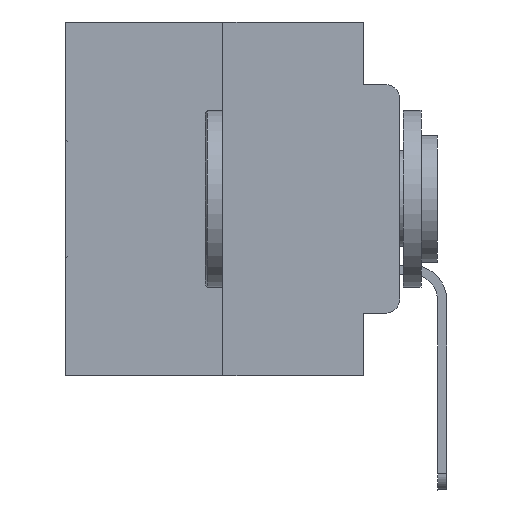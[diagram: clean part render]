
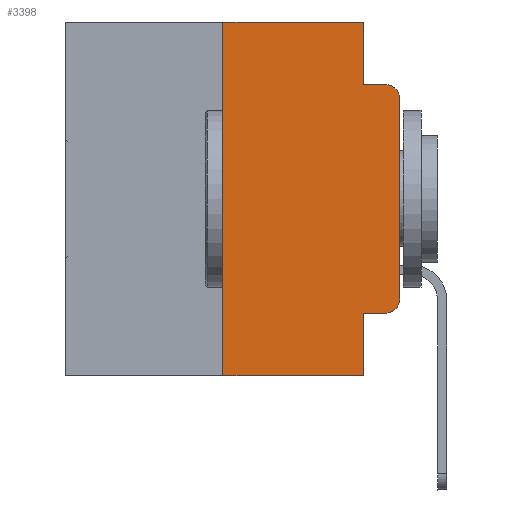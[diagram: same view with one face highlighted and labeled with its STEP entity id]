
A CAD part, left-side view. The second image highlights one B-rep face of the part: STEP entity #3398.
In plain terms, the highlighted planar face has unit normal (-1, 0, 0).
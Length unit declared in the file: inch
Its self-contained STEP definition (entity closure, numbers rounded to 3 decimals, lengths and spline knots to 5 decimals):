
#674 = DIRECTION ( 'NONE',  ( -1., 0., 0. ) ) ;
#1732 = EDGE_CURVE ( 'NONE', #10366, #27872, #18274, .T. ) ;
#1912 = VERTEX_POINT ( 'NONE', #21040 ) ;
#2130 = EDGE_CURVE ( 'NONE', #7641, #21543, #20553, .T. ) ;
#2173 = DIRECTION ( 'NONE',  ( 0., 0., -1. ) ) ;
#2316 = CARTESIAN_POINT ( 'NONE',  ( 0., 0.473, 0. ) ) ;
#2382 = VECTOR ( 'NONE', #18205, 39.37008 ) ;
#2427 = ORIENTED_EDGE ( 'NONE', *, *, #14850, .F. ) ;
#2799 = ORIENTED_EDGE ( 'NONE', *, *, #20841, .T. ) ;
#3170 = AXIS2_PLACEMENT_3D ( 'NONE', #11719, #674, #25266 ) ;
#3317 = CARTESIAN_POINT ( 'NONE',  ( 0., 0., 0. ) ) ;
#3398 = ADVANCED_FACE ( 'NONE', ( #11137 ), #13498, .F. ) ;
#4676 = EDGE_CURVE ( 'NONE', #13734, #19552, #22344, .T. ) ;
#5576 = ORIENTED_EDGE ( 'NONE', *, *, #4676, .F. ) ;
#5836 = VERTEX_POINT ( 'NONE', #7557 ) ;
#6336 = CARTESIAN_POINT ( 'NONE',  ( 0., 0.051, 0. ) ) ;
#6423 = DIRECTION ( 'NONE',  ( 0., -1., 0. ) ) ;
#6621 = CARTESIAN_POINT ( 'NONE',  ( 0., 0.02, -0.1085 ) ) ;
#6724 = CARTESIAN_POINT ( 'NONE',  ( 0., 0.25, 0. ) ) ;
#6899 = DIRECTION ( 'NONE',  ( -1., 0., 0. ) ) ;
#7078 = DIRECTION ( 'NONE',  ( 0., -1., 0. ) ) ;
#7557 = CARTESIAN_POINT ( 'NONE',  ( 0., 0., -0.3915 ) ) ;
#7641 = VERTEX_POINT ( 'NONE', #23412 ) ;
#7825 = LINE ( 'NONE', #10033, #12091 ) ;
#9768 = CARTESIAN_POINT ( 'NONE',  ( 0., 0., -0.1085 ) ) ;
#9896 = DIRECTION ( 'NONE',  ( 0., 0., -1. ) ) ;
#10033 = CARTESIAN_POINT ( 'NONE',  ( 0., 0.051, 0. ) ) ;
#10095 = ORIENTED_EDGE ( 'NONE', *, *, #27445, .F. ) ;
#10366 = VERTEX_POINT ( 'NONE', #9768 ) ;
#11137 = FACE_OUTER_BOUND ( 'NONE', #25460, .T. ) ;
#11202 = VECTOR ( 'NONE', #6423, 39.37008 ) ;
#11481 = CARTESIAN_POINT ( 'NONE',  ( 0., 0.473, -0.5 ) ) ;
#11497 = CARTESIAN_POINT ( 'NONE',  ( 0., 0.25, 0. ) ) ;
#11633 = CARTESIAN_POINT ( 'NONE',  ( 0., 0.051, -0.0885 ) ) ;
#11719 = CARTESIAN_POINT ( 'NONE',  ( 0., 0.02, -0.3915 ) ) ;
#11766 = CARTESIAN_POINT ( 'NONE',  ( 0., 0.051, -0.4115 ) ) ;
#12091 = VECTOR ( 'NONE', #9896, 39.37008 ) ;
#13355 = DIRECTION ( 'NONE',  ( 0., 0., -1. ) ) ;
#13498 = PLANE ( 'NONE',  #20268 ) ;
#13734 = VERTEX_POINT ( 'NONE', #15559 ) ;
#13778 = EDGE_CURVE ( 'NONE', #1912, #5836, #20082, .T. ) ;
#13835 = ORIENTED_EDGE ( 'NONE', *, *, #24456, .T. ) ;
#14768 = DIRECTION ( 'NONE',  ( 0., 0., 1. ) ) ;
#14850 = EDGE_CURVE ( 'NONE', #21543, #27362, #27032, .T. ) ;
#15559 = CARTESIAN_POINT ( 'NONE',  ( 0., 0.051, -0.4115 ) ) ;
#15654 = ORIENTED_EDGE ( 'NONE', *, *, #25954, .F. ) ;
#15881 = LINE ( 'NONE', #11766, #17844 ) ;
#16478 = DIRECTION ( 'NONE',  ( 0., -1., 0. ) ) ;
#16547 = ORIENTED_EDGE ( 'NONE', *, *, #13778, .T. ) ;
#16866 = VECTOR ( 'NONE', #20192, 39.37008 ) ;
#17844 = VECTOR ( 'NONE', #16478, 39.37008 ) ;
#18205 = DIRECTION ( 'NONE',  ( 0., 0., 1. ) ) ;
#18213 = CARTESIAN_POINT ( 'NONE',  ( 0., 0.473, 0. ) ) ;
#18274 = CIRCLE ( 'NONE', #27205, 0.02 ) ;
#18275 = LINE ( 'NONE', #11633, #16866 ) ;
#19164 = VECTOR ( 'NONE', #14768, 39.37008 ) ;
#19552 = VERTEX_POINT ( 'NONE', #25103 ) ;
#20026 = LINE ( 'NONE', #11481, #22937 ) ;
#20082 = CIRCLE ( 'NONE', #3170, 0.02 ) ;
#20107 = ORIENTED_EDGE ( 'NONE', *, *, #1732, .T. ) ;
#20192 = DIRECTION ( 'NONE',  ( 0., -1., 0. ) ) ;
#20268 = AXIS2_PLACEMENT_3D ( 'NONE', #18213, #22489, #13355 ) ;
#20553 = LINE ( 'NONE', #6724, #2382 ) ;
#20782 = ORIENTED_EDGE ( 'NONE', *, *, #26196, .T. ) ;
#20841 = EDGE_CURVE ( 'NONE', #13734, #1912, #15881, .T. ) ;
#20945 = CARTESIAN_POINT ( 'NONE',  ( 0., 0.051, -0.0885 ) ) ;
#21040 = CARTESIAN_POINT ( 'NONE',  ( 0., 0.02, -0.4115 ) ) ;
#21543 = VERTEX_POINT ( 'NONE', #11497 ) ;
#21691 = ORIENTED_EDGE ( 'NONE', *, *, #2130, .F. ) ;
#21905 = CARTESIAN_POINT ( 'NONE',  ( 0., 0.051, 0. ) ) ;
#22344 = LINE ( 'NONE', #21905, #24574 ) ;
#22489 = DIRECTION ( 'NONE',  ( 1., 0., 0. ) ) ;
#22937 = VECTOR ( 'NONE', #7078, 39.37008 ) ;
#23412 = CARTESIAN_POINT ( 'NONE',  ( 0., 0.25, -0.5 ) ) ;
#23478 = LINE ( 'NONE', #3317, #19164 ) ;
#24456 = EDGE_CURVE ( 'NONE', #5836, #10366, #23478, .T. ) ;
#24574 = VECTOR ( 'NONE', #2173, 39.37008 ) ;
#25103 = CARTESIAN_POINT ( 'NONE',  ( 0., 0.051, -0.5 ) ) ;
#25266 = DIRECTION ( 'NONE',  ( 0., 0., -1. ) ) ;
#25460 = EDGE_LOOP ( 'NONE', ( #13835, #20107, #10095, #15654, #2427, #21691, #20782, #5576, #2799, #16547 ) ) ;
#25954 = EDGE_CURVE ( 'NONE', #27362, #27181, #7825, .T. ) ;
#26059 = CARTESIAN_POINT ( 'NONE',  ( 0., 0.02, -0.0885 ) ) ;
#26196 = EDGE_CURVE ( 'NONE', #7641, #19552, #20026, .T. ) ;
#26940 = DIRECTION ( 'NONE',  ( 0., 0., -1. ) ) ;
#27032 = LINE ( 'NONE', #2316, #11202 ) ;
#27181 = VERTEX_POINT ( 'NONE', #20945 ) ;
#27205 = AXIS2_PLACEMENT_3D ( 'NONE', #6621, #6899, #26940 ) ;
#27362 = VERTEX_POINT ( 'NONE', #6336 ) ;
#27445 = EDGE_CURVE ( 'NONE', #27181, #27872, #18275, .T. ) ;
#27872 = VERTEX_POINT ( 'NONE', #26059 ) ;
